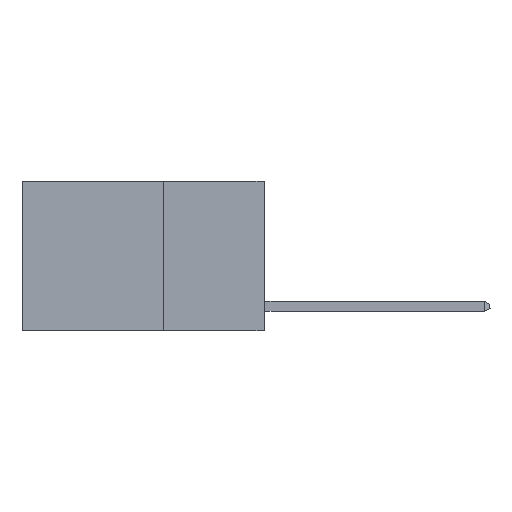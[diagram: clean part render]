
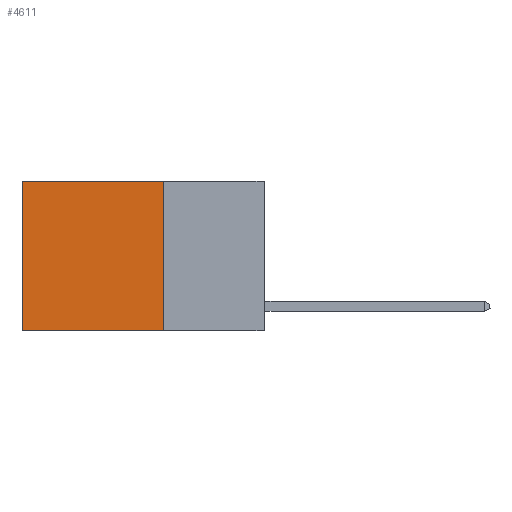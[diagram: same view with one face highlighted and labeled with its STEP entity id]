
A CAD part, left-side view. The second image highlights one B-rep face of the part: STEP entity #4611.
In plain terms, the highlighted planar face has unit normal (-1, 0, 0).
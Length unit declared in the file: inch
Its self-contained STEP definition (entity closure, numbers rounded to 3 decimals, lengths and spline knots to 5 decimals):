
#6 = CARTESIAN_POINT ( 'NONE',  ( 0.2625, 0.25, 0. ) ) ;
#291 = LINE ( 'NONE', #12034, #11031 ) ;
#461 = EDGE_CURVE ( 'NONE', #3618, #2802, #5202, .T. ) ;
#552 = ORIENTED_EDGE ( 'NONE', *, *, #3635, .T. ) ;
#1219 = DIRECTION ( 'NONE',  ( 0., 0., -1. ) ) ;
#1228 = EDGE_LOOP ( 'NONE', ( #10039, #3529, #13705, #552 ) ) ;
#1354 = AXIS2_PLACEMENT_3D ( 'NONE', #6, #9850, #3742 ) ;
#1611 = DIRECTION ( 'NONE',  ( 0., 1., 0. ) ) ;
#2431 = CARTESIAN_POINT ( 'NONE',  ( 0.2625, 0.25, -0.37 ) ) ;
#2527 = VECTOR ( 'NONE', #1219, 39.37008 ) ;
#2802 = VERTEX_POINT ( 'NONE', #9568 ) ;
#3529 = ORIENTED_EDGE ( 'NONE', *, *, #6260, .F. ) ;
#3618 = VERTEX_POINT ( 'NONE', #13272 ) ;
#3635 = EDGE_CURVE ( 'NONE', #10688, #3618, #291, .T. ) ;
#3742 = DIRECTION ( 'NONE',  ( 0., 0., -1. ) ) ;
#4611 = ADVANCED_FACE ( 'NONE', ( #15686 ), #7326, .F. ) ;
#5202 = LINE ( 'NONE', #7602, #2527 ) ;
#6260 = EDGE_CURVE ( 'NONE', #9550, #2802, #7369, .T. ) ;
#6357 = CARTESIAN_POINT ( 'NONE',  ( 0.2625, 0.25, -0.37 ) ) ;
#6862 = VECTOR ( 'NONE', #7909, 39.37008 ) ;
#7193 = DIRECTION ( 'NONE',  ( 0., 1., 0. ) ) ;
#7326 = PLANE ( 'NONE',  #1354 ) ;
#7369 = LINE ( 'NONE', #6357, #15577 ) ;
#7602 = CARTESIAN_POINT ( 'NONE',  ( 0.2625, 0.6, 0. ) ) ;
#7909 = DIRECTION ( 'NONE',  ( 0., 0., -1. ) ) ;
#9550 = VERTEX_POINT ( 'NONE', #2431 ) ;
#9568 = CARTESIAN_POINT ( 'NONE',  ( 0.2625, 0.6, -0.37 ) ) ;
#9807 = EDGE_CURVE ( 'NONE', #10688, #9550, #13527, .T. ) ;
#9850 = DIRECTION ( 'NONE',  ( 1., 0., 0. ) ) ;
#10039 = ORIENTED_EDGE ( 'NONE', *, *, #461, .T. ) ;
#10096 = CARTESIAN_POINT ( 'NONE',  ( 0.2625, 0.25, 0. ) ) ;
#10688 = VERTEX_POINT ( 'NONE', #14264 ) ;
#11031 = VECTOR ( 'NONE', #7193, 39.37008 ) ;
#12034 = CARTESIAN_POINT ( 'NONE',  ( 0.2625, 0.25, 0. ) ) ;
#13272 = CARTESIAN_POINT ( 'NONE',  ( 0.2625, 0.6, 0. ) ) ;
#13527 = LINE ( 'NONE', #10096, #6862 ) ;
#13705 = ORIENTED_EDGE ( 'NONE', *, *, #9807, .F. ) ;
#14264 = CARTESIAN_POINT ( 'NONE',  ( 0.2625, 0.25, 0. ) ) ;
#15577 = VECTOR ( 'NONE', #1611, 39.37008 ) ;
#15686 = FACE_OUTER_BOUND ( 'NONE', #1228, .T. ) ;
